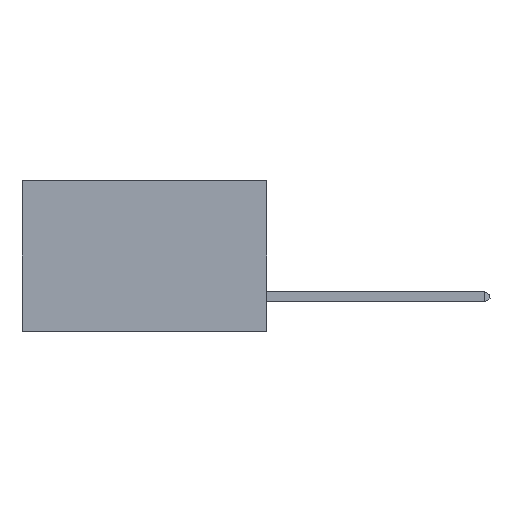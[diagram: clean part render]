
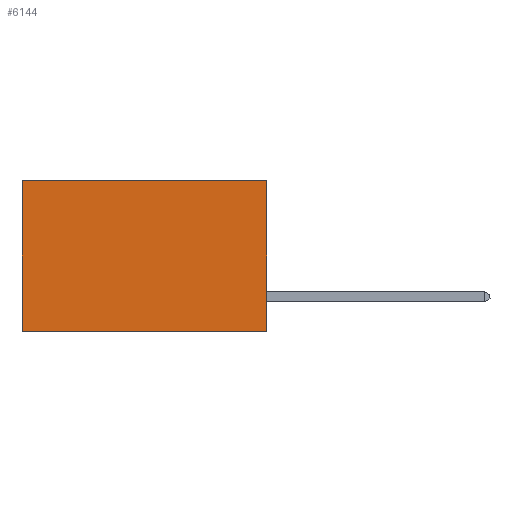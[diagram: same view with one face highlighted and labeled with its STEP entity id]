
A CAD part, left-side view. The second image highlights one B-rep face of the part: STEP entity #6144.
In plain terms, the highlighted planar face has unit normal (-1, 0, 0).
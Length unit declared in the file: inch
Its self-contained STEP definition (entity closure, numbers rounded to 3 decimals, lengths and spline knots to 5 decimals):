
#210 = CARTESIAN_POINT ( 'NONE',  ( 0.2875, 0., -0.37 ) ) ;
#1134 = VERTEX_POINT ( 'NONE', #210 ) ;
#1808 = LINE ( 'NONE', #3053, #10919 ) ;
#1855 = EDGE_CURVE ( 'NONE', #12192, #6867, #14433, .T. ) ;
#3053 = CARTESIAN_POINT ( 'NONE',  ( 0.2875, 0.6, 0. ) ) ;
#3196 = DIRECTION ( 'NONE',  ( 0., 0., -1. ) ) ;
#3234 = VERTEX_POINT ( 'NONE', #3802 ) ;
#3588 = VECTOR ( 'NONE', #12858, 39.37008 ) ;
#3605 = CARTESIAN_POINT ( 'NONE',  ( 0.2875, 0., 0. ) ) ;
#3734 = LINE ( 'NONE', #7307, #9306 ) ;
#3802 = CARTESIAN_POINT ( 'NONE',  ( 0.2875, 0.6, -0.37 ) ) ;
#3932 = EDGE_CURVE ( 'NONE', #12192, #1134, #3734, .T. ) ;
#3984 = LINE ( 'NONE', #11692, #3588 ) ;
#4284 = DIRECTION ( 'NONE',  ( 0., 0., -1. ) ) ;
#5964 = FACE_OUTER_BOUND ( 'NONE', #6019, .T. ) ;
#6019 = EDGE_LOOP ( 'NONE', ( #14040, #14218, #15297, #14524 ) ) ;
#6144 = ADVANCED_FACE ( 'NONE', ( #5964 ), #8866, .F. ) ;
#6867 = VERTEX_POINT ( 'NONE', #9742 ) ;
#7307 = CARTESIAN_POINT ( 'NONE',  ( 0.2875, 0., 0. ) ) ;
#8370 = EDGE_CURVE ( 'NONE', #6867, #3234, #1808, .T. ) ;
#8650 = VECTOR ( 'NONE', #13789, 39.37008 ) ;
#8847 = DIRECTION ( 'NONE',  ( 1., 0., 0. ) ) ;
#8852 = CARTESIAN_POINT ( 'NONE',  ( 0.2875, 0., 0. ) ) ;
#8866 = PLANE ( 'NONE',  #9522 ) ;
#9306 = VECTOR ( 'NONE', #3196, 39.37008 ) ;
#9522 = AXIS2_PLACEMENT_3D ( 'NONE', #8852, #8847, #10022 ) ;
#9742 = CARTESIAN_POINT ( 'NONE',  ( 0.2875, 0.6, 0. ) ) ;
#10022 = DIRECTION ( 'NONE',  ( 0., 0., -1. ) ) ;
#10775 = EDGE_CURVE ( 'NONE', #1134, #3234, #3984, .T. ) ;
#10919 = VECTOR ( 'NONE', #4284, 39.37008 ) ;
#11692 = CARTESIAN_POINT ( 'NONE',  ( 0.2875, 0., -0.37 ) ) ;
#12192 = VERTEX_POINT ( 'NONE', #3605 ) ;
#12858 = DIRECTION ( 'NONE',  ( 0., 1., 0. ) ) ;
#13789 = DIRECTION ( 'NONE',  ( 0., 1., 0. ) ) ;
#14040 = ORIENTED_EDGE ( 'NONE', *, *, #8370, .T. ) ;
#14218 = ORIENTED_EDGE ( 'NONE', *, *, #10775, .F. ) ;
#14433 = LINE ( 'NONE', #14970, #8650 ) ;
#14524 = ORIENTED_EDGE ( 'NONE', *, *, #1855, .T. ) ;
#14970 = CARTESIAN_POINT ( 'NONE',  ( 0.2875, 0., 0. ) ) ;
#15297 = ORIENTED_EDGE ( 'NONE', *, *, #3932, .F. ) ;
